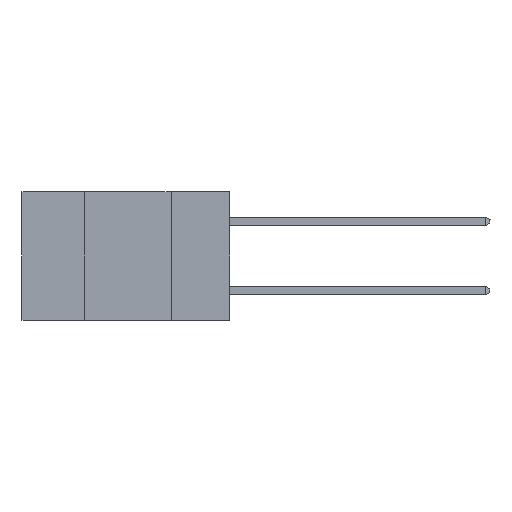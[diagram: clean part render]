
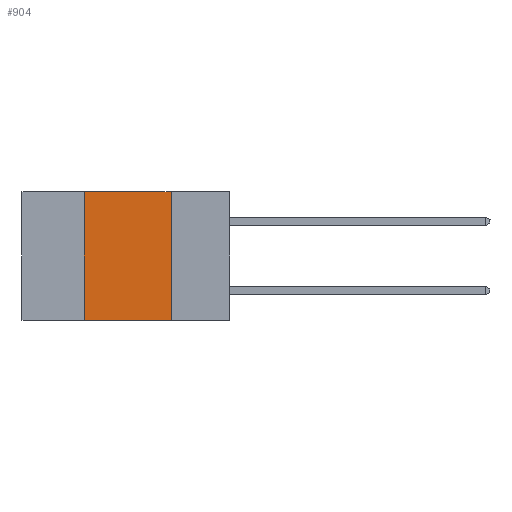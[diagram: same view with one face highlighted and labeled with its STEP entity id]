
A CAD part, left-side view. The second image highlights one B-rep face of the part: STEP entity #904.
In plain terms, the highlighted planar face has unit normal (-1, 0, 0).
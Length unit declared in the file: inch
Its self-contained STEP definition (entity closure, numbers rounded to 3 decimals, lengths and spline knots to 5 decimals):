
#246 = CARTESIAN_POINT ( 'NONE',  ( 0., 0.17, -0.37 ) ) ;
#904 = ADVANCED_FACE ( 'NONE', ( #2391 ), #3341, .F. ) ;
#1248 = CARTESIAN_POINT ( 'NONE',  ( 0., 0.42, 0. ) ) ;
#1557 = DIRECTION ( 'NONE',  ( 0., 0., -1. ) ) ;
#2010 = VERTEX_POINT ( 'NONE', #1248 ) ;
#2391 = FACE_OUTER_BOUND ( 'NONE', #9930, .T. ) ;
#2485 = ORIENTED_EDGE ( 'NONE', *, *, #10813, .F. ) ;
#2491 = DIRECTION ( 'NONE',  ( 0., -1., 0. ) ) ;
#3341 = PLANE ( 'NONE',  #9573 ) ;
#3503 = LINE ( 'NONE', #4407, #7689 ) ;
#4400 = EDGE_CURVE ( 'NONE', #11393, #6773, #6623, .T. ) ;
#4407 = CARTESIAN_POINT ( 'NONE',  ( 0., 0.6, -0.37 ) ) ;
#4617 = ORIENTED_EDGE ( 'NONE', *, *, #4400, .F. ) ;
#5157 = VECTOR ( 'NONE', #6005, 39.37008 ) ;
#5461 = EDGE_CURVE ( 'NONE', #8502, #6773, #3503, .T. ) ;
#6005 = DIRECTION ( 'NONE',  ( 0., 0., 1. ) ) ;
#6153 = ORIENTED_EDGE ( 'NONE', *, *, #5461, .T. ) ;
#6172 = CARTESIAN_POINT ( 'NONE',  ( 0., 0.17, -0.37 ) ) ;
#6234 = ORIENTED_EDGE ( 'NONE', *, *, #10999, .F. ) ;
#6623 = LINE ( 'NONE', #246, #11166 ) ;
#6773 = VERTEX_POINT ( 'NONE', #6172 ) ;
#7543 = DIRECTION ( 'NONE',  ( 0., 0., -1. ) ) ;
#7628 = LINE ( 'NONE', #8525, #5157 ) ;
#7689 = VECTOR ( 'NONE', #2491, 39.37008 ) ;
#7741 = CARTESIAN_POINT ( 'NONE',  ( 0., 0.6, 0. ) ) ;
#8502 = VERTEX_POINT ( 'NONE', #8815 ) ;
#8525 = CARTESIAN_POINT ( 'NONE',  ( 0., 0.42, -0.37 ) ) ;
#8739 = CARTESIAN_POINT ( 'NONE',  ( 0., 0.17, 0. ) ) ;
#8815 = CARTESIAN_POINT ( 'NONE',  ( 0., 0.42, -0.37 ) ) ;
#9081 = DIRECTION ( 'NONE',  ( 0., -1., 0. ) ) ;
#9409 = VECTOR ( 'NONE', #9081, 39.37008 ) ;
#9573 = AXIS2_PLACEMENT_3D ( 'NONE', #7741, #11437, #1557 ) ;
#9749 = LINE ( 'NONE', #10855, #9409 ) ;
#9930 = EDGE_LOOP ( 'NONE', ( #4617, #6234, #2485, #6153 ) ) ;
#10813 = EDGE_CURVE ( 'NONE', #8502, #2010, #7628, .T. ) ;
#10855 = CARTESIAN_POINT ( 'NONE',  ( 0., 0.6, 0. ) ) ;
#10999 = EDGE_CURVE ( 'NONE', #2010, #11393, #9749, .T. ) ;
#11166 = VECTOR ( 'NONE', #7543, 39.37008 ) ;
#11393 = VERTEX_POINT ( 'NONE', #8739 ) ;
#11437 = DIRECTION ( 'NONE',  ( 1., 0., 0. ) ) ;
